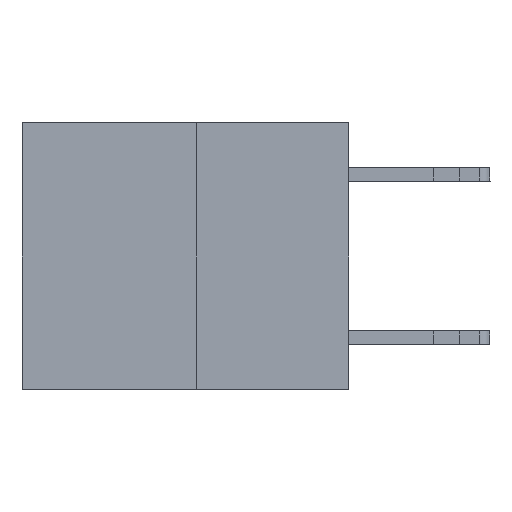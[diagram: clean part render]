
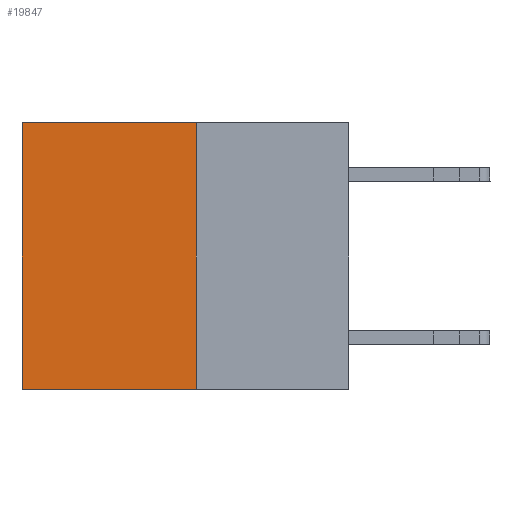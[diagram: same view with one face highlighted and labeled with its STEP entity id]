
A CAD part, left-side view. The second image highlights one B-rep face of the part: STEP entity #19847.
In plain terms, the highlighted planar face has unit normal (-1, 0, 0).
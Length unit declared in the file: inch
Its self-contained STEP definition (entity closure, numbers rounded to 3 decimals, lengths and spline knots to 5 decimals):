
#277 = VERTEX_POINT ( 'NONE', #11567 ) ;
#2827 = CARTESIAN_POINT ( 'NONE',  ( 0.3165, 0.6, 0. ) ) ;
#3239 = VECTOR ( 'NONE', #4810, 39.37008 ) ;
#4810 = DIRECTION ( 'NONE',  ( 0., 0., -1. ) ) ;
#4925 = CARTESIAN_POINT ( 'NONE',  ( 0.3165, 0.6, -0.49 ) ) ;
#6904 = LINE ( 'NONE', #25930, #3239 ) ;
#7494 = FACE_OUTER_BOUND ( 'NONE', #26395, .T. ) ;
#7547 = CARTESIAN_POINT ( 'NONE',  ( 0.3165, 0.28, -0.49 ) ) ;
#7564 = ORIENTED_EDGE ( 'NONE', *, *, #24573, .T. ) ;
#7961 = CARTESIAN_POINT ( 'NONE',  ( 0.3165, 0.28, -0.49 ) ) ;
#8045 = DIRECTION ( 'NONE',  ( 0., 0., -1. ) ) ;
#8237 = EDGE_CURVE ( 'NONE', #21429, #277, #20251, .T. ) ;
#8964 = VECTOR ( 'NONE', #23848, 39.37008 ) ;
#10059 = DIRECTION ( 'NONE',  ( 1., 0., 0. ) ) ;
#10632 = DIRECTION ( 'NONE',  ( 0., 0., -1. ) ) ;
#11567 = CARTESIAN_POINT ( 'NONE',  ( 0.3165, 0.28, -0.49 ) ) ;
#12276 = VECTOR ( 'NONE', #10632, 39.37008 ) ;
#12449 = AXIS2_PLACEMENT_3D ( 'NONE', #7961, #10059, #8045 ) ;
#12528 = ORIENTED_EDGE ( 'NONE', *, *, #22744, .T. ) ;
#15235 = LINE ( 'NONE', #24227, #8964 ) ;
#15761 = VERTEX_POINT ( 'NONE', #4925 ) ;
#16100 = VECTOR ( 'NONE', #26954, 39.37008 ) ;
#16653 = PLANE ( 'NONE',  #12449 ) ;
#19847 = ADVANCED_FACE ( 'NONE', ( #7494 ), #16653, .F. ) ;
#20251 = LINE ( 'NONE', #21404, #12276 ) ;
#21404 = CARTESIAN_POINT ( 'NONE',  ( 0.3165, 0.28, -0.49 ) ) ;
#21429 = VERTEX_POINT ( 'NONE', #22452 ) ;
#22452 = CARTESIAN_POINT ( 'NONE',  ( 0.3165, 0.28, 0. ) ) ;
#22744 = EDGE_CURVE ( 'NONE', #21429, #26251, #15235, .T. ) ;
#23848 = DIRECTION ( 'NONE',  ( 0., 1., 0. ) ) ;
#24227 = CARTESIAN_POINT ( 'NONE',  ( 0.3165, 0.28, 0. ) ) ;
#24387 = LINE ( 'NONE', #7547, #16100 ) ;
#24573 = EDGE_CURVE ( 'NONE', #26251, #15761, #6904, .T. ) ;
#24695 = ORIENTED_EDGE ( 'NONE', *, *, #25783, .F. ) ;
#25688 = ORIENTED_EDGE ( 'NONE', *, *, #8237, .F. ) ;
#25783 = EDGE_CURVE ( 'NONE', #277, #15761, #24387, .T. ) ;
#25930 = CARTESIAN_POINT ( 'NONE',  ( 0.3165, 0.6, -0.49 ) ) ;
#26251 = VERTEX_POINT ( 'NONE', #2827 ) ;
#26395 = EDGE_LOOP ( 'NONE', ( #7564, #24695, #25688, #12528 ) ) ;
#26954 = DIRECTION ( 'NONE',  ( 0., 1., 0. ) ) ;
